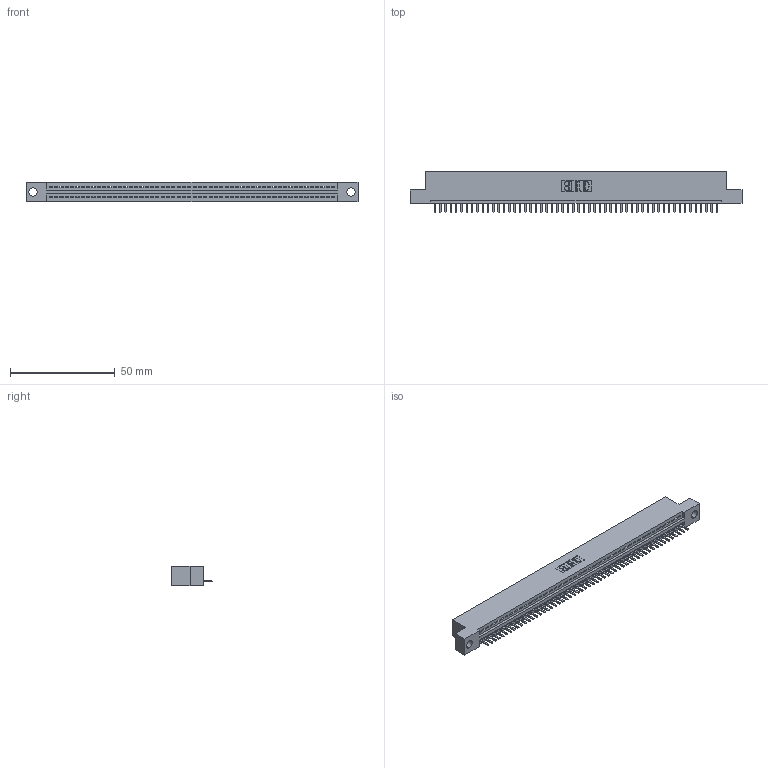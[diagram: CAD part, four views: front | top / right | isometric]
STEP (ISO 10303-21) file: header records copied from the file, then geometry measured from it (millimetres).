
FILE_DESCRIPTION (( 'STEP AP203' ), '1' );
FILE_NAME ('395-054-520-104.STEP', '2021-05-31T21:32:21', ( '' ), ( '' ), 'SwSTEP 2.0', 'SolidWorks 2020', '' );
FILE_SCHEMA (( 'CONFIG_CONTROL_DESIGN' ));
Length unit declared in the file: inch
Products named in the file (3): 345 Part_Flush Mounting Lugs - 0.156 Dia-TI; 345-292-001_345-293-120; 395-054-520-104
Assembly tree (55 placements, depth 2):
  395-054-520-104
    345 Part_Flush Mounting Lugs - 0.156 Dia-TI
    345-292-001_345-293-120  x54
Bounding box: 158.37 x 19.68 x 9.4 mm (x, y, z)
Volume: 14879.1 mm3; surface area: 19270.3 mm2
Topology: 55 solids, 55 shells, 3488 faces, 10313 edges, 6730 vertices
Faces by surface type: plane 2362, cylinder 1126
Entity records: 39559 total; most frequent: CARTESIAN_POINT 6872, ORIENTED_EDGE 6846, DIRECTION 5971, EDGE_CURVE 3423, LINE 3071, VECTOR 3071, VERTEX_POINT 2278, AXIS2_PLACEMENT_3D 1450
